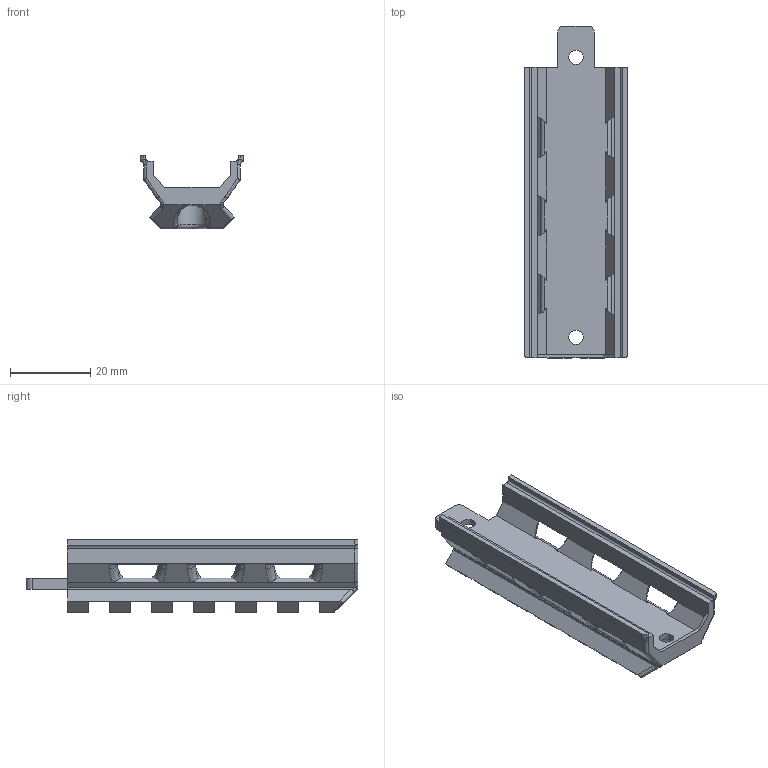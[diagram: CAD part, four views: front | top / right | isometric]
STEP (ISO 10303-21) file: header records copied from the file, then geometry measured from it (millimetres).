
FILE_DESCRIPTION(/* description */ (''),/* implementation_level */ '2;1');
FILE_NAME(/* name */ 'Picatinny Replacement Rail v7.step',/* time_stamp */ '2020-06-28T23:47:41-04:00',/* author */ (''),/* organization */ (''),/* preprocessor_version */ 'ST-DEVELOPER v18.1',/* originating_system */ 'Autodesk Translation Framework v9.3.0.1241',/* authorisation */ '');
FILE_SCHEMA (('AUTOMOTIVE_DESIGN { 1 0 10303 214 3 1 1 }'));
Length unit declared in the file: millimetre
Products named in the file (2): Picatinny Replacement Rail; Plate
Assembly tree (1 placements, depth 2):
  Picatinny Replacement Rail
    Plate
Bounding box: 25.65 x 82.7 x 18.34 mm (x, y, z)
Volume: 11662.2 mm3; surface area: 8382.9 mm2
Topology: 1 solids, 1 shells, 189 faces, 565 edges, 364 vertices
Faces by surface type: plane 98, cylinder 58, bspline 29, torus 4
Full cylindrical faces by diameter (mm): 3.55 x2, 7.2 x2
Entity records: 7292 total; most frequent: CARTESIAN_POINT 2281, ORIENTED_EDGE 1126, DIRECTION 947, EDGE_CURVE 563, VERTEX_POINT 364, AXIS2_PLACEMENT_3D 319, LINE 309, VECTOR 309
